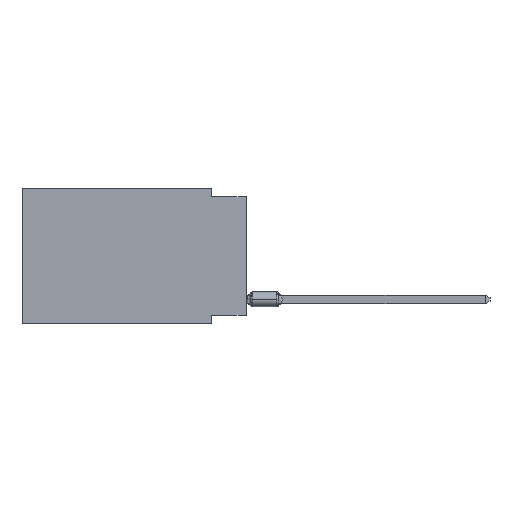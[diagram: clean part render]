
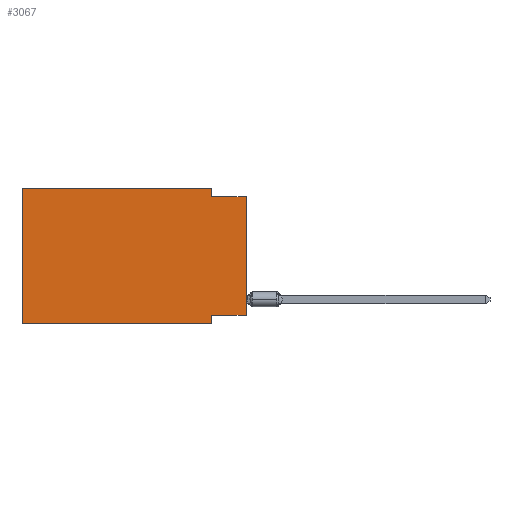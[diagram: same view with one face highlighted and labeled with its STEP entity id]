
A CAD part, left-side view. The second image highlights one B-rep face of the part: STEP entity #3067.
In plain terms, the highlighted planar face has unit normal (-1, 0, 0).
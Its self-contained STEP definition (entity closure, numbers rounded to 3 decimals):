
#225 = AXIS2_PLACEMENT_3D ( 'NONE', #2067, #9205, #6786 ) ;
#286 = VECTOR ( 'NONE', #5754, 1000. ) ;
#458 = VECTOR ( 'NONE', #5361, 1000. ) ;
#729 = VECTOR ( 'NONE', #1492, 1000. ) ;
#1492 = DIRECTION ( 'NONE',  ( 0., -1., 0. ) ) ;
#1566 = CARTESIAN_POINT ( 'NONE',  ( 0., 16.383, -9.906 ) ) ;
#1810 = CARTESIAN_POINT ( 'NONE',  ( 0., 16.383, 0. ) ) ;
#2067 = CARTESIAN_POINT ( 'NONE',  ( 0., 16.383, 0. ) ) ;
#2243 = CARTESIAN_POINT ( 'NONE',  ( 0., 0., -0.635 ) ) ;
#2255 = EDGE_CURVE ( 'NONE', #5668, #14976, #9031, .T. ) ;
#2304 = CARTESIAN_POINT ( 'NONE',  ( 0., 2.54, 0. ) ) ;
#3028 = DIRECTION ( 'NONE',  ( 0., 0., -1. ) ) ;
#3047 = DIRECTION ( 'NONE',  ( 0., 0., 1. ) ) ;
#3067 = ADVANCED_FACE ( 'NONE', ( #4338 ), #4645, .F. ) ;
#3126 = CARTESIAN_POINT ( 'NONE',  ( 0., 16.383, -9.906 ) ) ;
#3147 = VECTOR ( 'NONE', #3028, 1000. ) ;
#3454 = DIRECTION ( 'NONE',  ( 0., 1., 0. ) ) ;
#3843 = EDGE_CURVE ( 'NONE', #13374, #14976, #5230, .T. ) ;
#3900 = ORIENTED_EDGE ( 'NONE', *, *, #12765, .T. ) ;
#4302 = CARTESIAN_POINT ( 'NONE',  ( 0., 0., 0. ) ) ;
#4338 = FACE_OUTER_BOUND ( 'NONE', #12077, .T. ) ;
#4476 = LINE ( 'NONE', #14086, #9237 ) ;
#4645 = PLANE ( 'NONE',  #225 ) ;
#4951 = ORIENTED_EDGE ( 'NONE', *, *, #15392, .F. ) ;
#4997 = ORIENTED_EDGE ( 'NONE', *, *, #6900, .F. ) ;
#5001 = VERTEX_POINT ( 'NONE', #2304 ) ;
#5230 = LINE ( 'NONE', #10023, #3147 ) ;
#5361 = DIRECTION ( 'NONE',  ( 0., 0., -1. ) ) ;
#5668 = VERTEX_POINT ( 'NONE', #1566 ) ;
#5754 = DIRECTION ( 'NONE',  ( 0., -1., 0. ) ) ;
#6262 = ORIENTED_EDGE ( 'NONE', *, *, #10149, .F. ) ;
#6428 = CARTESIAN_POINT ( 'NONE',  ( 0., 2.54, -0.635 ) ) ;
#6667 = LINE ( 'NONE', #4302, #9995 ) ;
#6786 = DIRECTION ( 'NONE',  ( 0., 0., -1. ) ) ;
#6900 = EDGE_CURVE ( 'NONE', #5668, #15318, #15532, .T. ) ;
#7634 = LINE ( 'NONE', #7798, #458 ) ;
#7798 = CARTESIAN_POINT ( 'NONE',  ( 0., 2.54, 0. ) ) ;
#7977 = EDGE_CURVE ( 'NONE', #15318, #5001, #13755, .T. ) ;
#8030 = CARTESIAN_POINT ( 'NONE',  ( 0., 16.383, 0. ) ) ;
#8077 = CARTESIAN_POINT ( 'NONE',  ( 0., 16.383, 0. ) ) ;
#8215 = CARTESIAN_POINT ( 'NONE',  ( 0., 2.54, -9.271 ) ) ;
#8392 = CARTESIAN_POINT ( 'NONE',  ( 0., 0., -0.635 ) ) ;
#8472 = LINE ( 'NONE', #8392, #286 ) ;
#8787 = CARTESIAN_POINT ( 'NONE',  ( 0., 0., -9.271 ) ) ;
#9031 = LINE ( 'NONE', #3126, #14737 ) ;
#9177 = VERTEX_POINT ( 'NONE', #8787 ) ;
#9205 = DIRECTION ( 'NONE',  ( 1., 0., 0. ) ) ;
#9237 = VECTOR ( 'NONE', #3454, 1000. ) ;
#9995 = VECTOR ( 'NONE', #3047, 1000. ) ;
#10023 = CARTESIAN_POINT ( 'NONE',  ( 0., 2.54, -9.906 ) ) ;
#10149 = EDGE_CURVE ( 'NONE', #13896, #14573, #8472, .T. ) ;
#10499 = ORIENTED_EDGE ( 'NONE', *, *, #15223, .F. ) ;
#10713 = CARTESIAN_POINT ( 'NONE',  ( 0., 2.54, -9.906 ) ) ;
#11344 = ORIENTED_EDGE ( 'NONE', *, *, #3843, .F. ) ;
#11392 = ORIENTED_EDGE ( 'NONE', *, *, #2255, .T. ) ;
#12077 = EDGE_LOOP ( 'NONE', ( #3900, #6262, #10499, #15297, #4997, #11392, #11344, #4951 ) ) ;
#12625 = VECTOR ( 'NONE', #13103, 1000. ) ;
#12721 = DIRECTION ( 'NONE',  ( 0., -1., 0. ) ) ;
#12765 = EDGE_CURVE ( 'NONE', #9177, #14573, #6667, .T. ) ;
#13103 = DIRECTION ( 'NONE',  ( 0., 0., 1. ) ) ;
#13374 = VERTEX_POINT ( 'NONE', #8215 ) ;
#13755 = LINE ( 'NONE', #1810, #729 ) ;
#13896 = VERTEX_POINT ( 'NONE', #6428 ) ;
#14086 = CARTESIAN_POINT ( 'NONE',  ( 0., 0., -9.271 ) ) ;
#14573 = VERTEX_POINT ( 'NONE', #2243 ) ;
#14737 = VECTOR ( 'NONE', #12721, 1000. ) ;
#14976 = VERTEX_POINT ( 'NONE', #10713 ) ;
#15223 = EDGE_CURVE ( 'NONE', #5001, #13896, #7634, .T. ) ;
#15297 = ORIENTED_EDGE ( 'NONE', *, *, #7977, .F. ) ;
#15318 = VERTEX_POINT ( 'NONE', #8030 ) ;
#15392 = EDGE_CURVE ( 'NONE', #9177, #13374, #4476, .T. ) ;
#15532 = LINE ( 'NONE', #8077, #12625 ) ;
